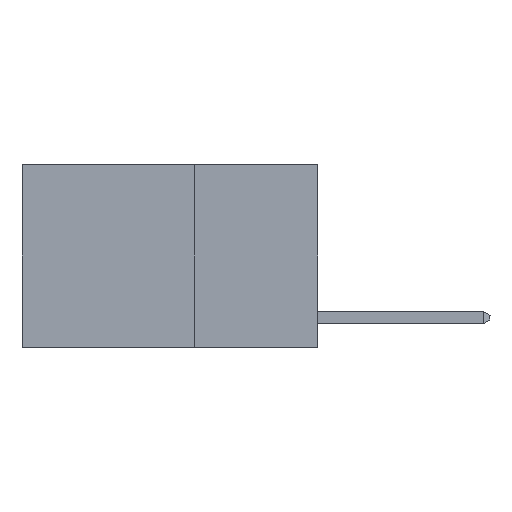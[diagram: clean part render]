
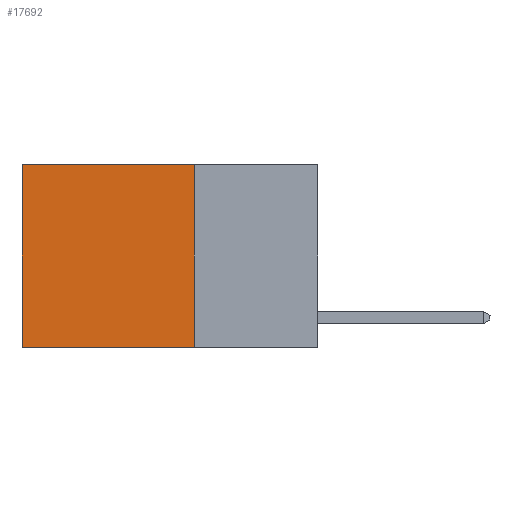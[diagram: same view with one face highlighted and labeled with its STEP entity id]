
A CAD part, left-side view. The second image highlights one B-rep face of the part: STEP entity #17692.
In plain terms, the highlighted planar face has unit normal (-1, 0, 0).
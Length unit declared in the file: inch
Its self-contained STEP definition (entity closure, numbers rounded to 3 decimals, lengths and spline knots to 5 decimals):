
#423 = DIRECTION ( 'NONE',  ( 0., 0., -1. ) ) ;
#1079 = VECTOR ( 'NONE', #4276, 39.37008 ) ;
#1583 = PLANE ( 'NONE',  #17424 ) ;
#2020 = VECTOR ( 'NONE', #3658, 39.37008 ) ;
#2602 = EDGE_LOOP ( 'NONE', ( #8328, #4997, #11614, #18103 ) ) ;
#3523 = CARTESIAN_POINT ( 'NONE',  ( 0.2625, 0.6, 0. ) ) ;
#3658 = DIRECTION ( 'NONE',  ( 0., 1., 0. ) ) ;
#4276 = DIRECTION ( 'NONE',  ( 0., 1., 0. ) ) ;
#4645 = VERTEX_POINT ( 'NONE', #11085 ) ;
#4997 = ORIENTED_EDGE ( 'NONE', *, *, #7662, .F. ) ;
#6261 = CARTESIAN_POINT ( 'NONE',  ( 0.2625, 0.25, 0. ) ) ;
#6369 = CARTESIAN_POINT ( 'NONE',  ( 0.2625, 0.25, 0. ) ) ;
#7662 = EDGE_CURVE ( 'NONE', #12503, #4645, #16064, .T. ) ;
#8328 = ORIENTED_EDGE ( 'NONE', *, *, #13147, .T. ) ;
#8574 = CARTESIAN_POINT ( 'NONE',  ( 0.2625, 0.25, 0. ) ) ;
#9427 = EDGE_CURVE ( 'NONE', #18465, #12503, #16210, .T. ) ;
#11085 = CARTESIAN_POINT ( 'NONE',  ( 0.2625, 0.6, -0.37 ) ) ;
#11614 = ORIENTED_EDGE ( 'NONE', *, *, #9427, .F. ) ;
#11740 = DIRECTION ( 'NONE',  ( 1., 0., 0. ) ) ;
#12106 = CARTESIAN_POINT ( 'NONE',  ( 0.2625, 0.6, 0. ) ) ;
#12372 = VECTOR ( 'NONE', #16270, 39.37008 ) ;
#12503 = VERTEX_POINT ( 'NONE', #13616 ) ;
#13147 = EDGE_CURVE ( 'NONE', #15631, #4645, #16082, .T. ) ;
#13181 = DIRECTION ( 'NONE',  ( 0., 0., -1. ) ) ;
#13568 = LINE ( 'NONE', #6369, #2020 ) ;
#13616 = CARTESIAN_POINT ( 'NONE',  ( 0.2625, 0.25, -0.37 ) ) ;
#13657 = CARTESIAN_POINT ( 'NONE',  ( 0.2625, 0.25, 0. ) ) ;
#14155 = EDGE_CURVE ( 'NONE', #18465, #15631, #13568, .T. ) ;
#15631 = VERTEX_POINT ( 'NONE', #12106 ) ;
#15928 = CARTESIAN_POINT ( 'NONE',  ( 0.2625, 0.25, -0.37 ) ) ;
#16064 = LINE ( 'NONE', #15928, #1079 ) ;
#16082 = LINE ( 'NONE', #3523, #16765 ) ;
#16210 = LINE ( 'NONE', #6261, #12372 ) ;
#16270 = DIRECTION ( 'NONE',  ( 0., 0., -1. ) ) ;
#16610 = FACE_OUTER_BOUND ( 'NONE', #2602, .T. ) ;
#16765 = VECTOR ( 'NONE', #423, 39.37008 ) ;
#17424 = AXIS2_PLACEMENT_3D ( 'NONE', #8574, #11740, #13181 ) ;
#17692 = ADVANCED_FACE ( 'NONE', ( #16610 ), #1583, .F. ) ;
#18103 = ORIENTED_EDGE ( 'NONE', *, *, #14155, .T. ) ;
#18465 = VERTEX_POINT ( 'NONE', #13657 ) ;
